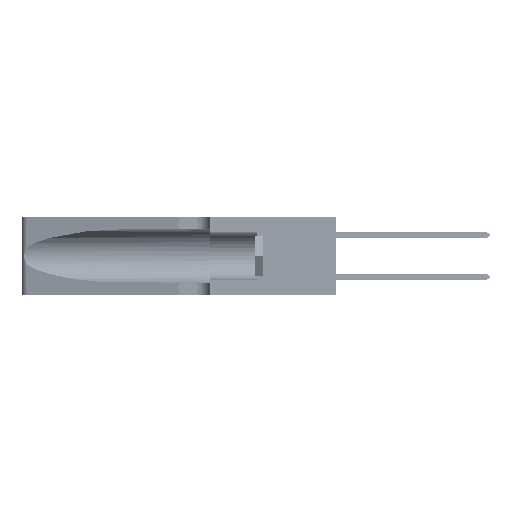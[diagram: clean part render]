
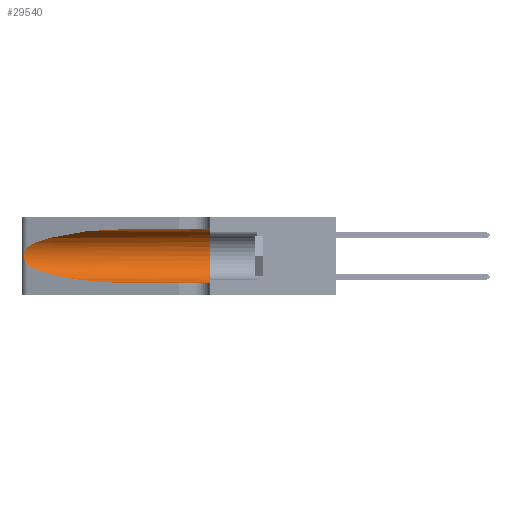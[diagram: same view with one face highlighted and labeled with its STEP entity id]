
A CAD part, left-side view. The second image highlights one B-rep face of the part: STEP entity #29540.
In plain terms, the highlighted cylindrical face has radius 3.308 mm (diameter 6.617 mm), a partial arc.
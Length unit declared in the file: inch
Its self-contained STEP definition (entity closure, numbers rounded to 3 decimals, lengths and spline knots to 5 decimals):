
#598 = FACE_OUTER_BOUND ( 'NONE', #2545, .T. ) ;
#1871 = ORIENTED_EDGE ( 'NONE', *, *, #4116, .T. ) ;
#2001 = CARTESIAN_POINT ( 'NONE',  ( 0.26075, 1.23896, 0.178 ) ) ;
#2328 = CARTESIAN_POINT ( 'NONE',  ( 0.25789, 1.23486, 0.15765 ) ) ;
#2545 = EDGE_LOOP ( 'NONE', ( #1871, #45478, #29068, #12682, #44403, #47040 ) ) ;
#3581 = B_SPLINE_CURVE_WITH_KNOTS ( 'NONE', 3,
 ( #9577, #37362, #22028, #49326, #21513, #45656, #10251, #2001, #37871, #29600, #2328, #5927, #49850, #9922 ),
 .UNSPECIFIED., .F., .F.,
 ( 4, 2, 2, 2, 2, 2, 4 ),
 ( 0., 0.00027, 0.00053, 0.00107, 0.0016, 0.00187, 0.00214 ),
 .UNSPECIFIED. ) ;
#4116 = EDGE_CURVE ( 'NONE', #36163, #9208, #4885, .T. ) ;
#4885 =( BOUNDED_CURVE ( )  B_SPLINE_CURVE ( 3, ( #5275, #32957, #40809, #21198 ),
 .UNSPECIFIED., .F., .F. ) 
 B_SPLINE_CURVE_WITH_KNOTS ( ( 4, 4 ),
 ( 1.5708, 2.84003 ),
 .UNSPECIFIED. ) 
 CURVE ( )  GEOMETRIC_REPRESENTATION_ITEM ( )  RATIONAL_B_SPLINE_CURVE ( ( 1., 0.87, 0.87, 1. ) ) 
 REPRESENTATION_ITEM ( '' )  );
#5275 = CARTESIAN_POINT ( 'NONE',  ( 0.1305, 0.72297, 0.31525 ) ) ;
#5927 = CARTESIAN_POINT ( 'NONE',  ( 0.25639, 1.23186, 0.15144 ) ) ;
#6183 = VECTOR ( 'NONE', #44947, 39.37008 ) ;
#6485 = DIRECTION ( 'NONE',  ( 0., -1., 0. ) ) ;
#7866 = CARTESIAN_POINT ( 'NONE',  ( 0.18966, 0.96281, 0.05475 ) ) ;
#7978 = DIRECTION ( 'NONE',  ( 0., 0., -1. ) ) ;
#8388 = CARTESIAN_POINT ( 'NONE',  ( 0.1305, 0.72297, 0.05475 ) ) ;
#8554 = CARTESIAN_POINT ( 'NONE',  ( 0.2373, 1.15595, 0.08982 ) ) ;
#9208 = VERTEX_POINT ( 'NONE', #44152 ) ;
#9269 = AXIS2_PLACEMENT_3D ( 'NONE', #34825, #50746, #35329 ) ;
#9577 = CARTESIAN_POINT ( 'NONE',  ( 0.25487, 1.22718, 0.22369 ) ) ;
#9922 = CARTESIAN_POINT ( 'NONE',  ( 0.25487, 1.22718, 0.14631 ) ) ;
#10251 = CARTESIAN_POINT ( 'NONE',  ( 0.26075, 1.23896, 0.19203 ) ) ;
#10557 = LINE ( 'NONE', #17931, #45785 ) ;
#12682 = ORIENTED_EDGE ( 'NONE', *, *, #26631, .T. ) ;
#16242 = CARTESIAN_POINT ( 'NONE',  ( 0.1305, 0.35, 0.05475 ) ) ;
#16866 = AXIS2_PLACEMENT_3D ( 'NONE', #23728, #47552, #7978 ) ;
#17245 = CARTESIAN_POINT ( 'NONE',  ( 0.1305, 0.35, 0.31525 ) ) ;
#17931 = CARTESIAN_POINT ( 'NONE',  ( 0.1305, 1.61858, 0.31525 ) ) ;
#19956 = EDGE_CURVE ( 'NONE', #27163, #28211, #43864, .T. ) ;
#20347 = CARTESIAN_POINT ( 'NONE',  ( 0.25487, 1.22718, 0.14631 ) ) ;
#21198 = CARTESIAN_POINT ( 'NONE',  ( 0.25487, 1.22718, 0.22369 ) ) ;
#21513 = CARTESIAN_POINT ( 'NONE',  ( 0.25854, 1.2359, 0.20912 ) ) ;
#22028 = CARTESIAN_POINT ( 'NONE',  ( 0.25639, 1.23184, 0.21858 ) ) ;
#22654 = VERTEX_POINT ( 'NONE', #30158 ) ;
#23728 = CARTESIAN_POINT ( 'NONE',  ( 0.1305, 1.61858, 0.185 ) ) ;
#26631 = EDGE_CURVE ( 'NONE', #33706, #28211, #37057, .T. ) ;
#27163 = VERTEX_POINT ( 'NONE', #17245 ) ;
#28211 = VERTEX_POINT ( 'NONE', #16242 ) ;
#29068 = ORIENTED_EDGE ( 'NONE', *, *, #49940, .T. ) ;
#29540 = ADVANCED_FACE ( 'NONE', ( #598 ), #35200, .F. ) ;
#29600 = CARTESIAN_POINT ( 'NONE',  ( 0.25856, 1.23593, 0.16098 ) ) ;
#30158 = CARTESIAN_POINT ( 'NONE',  ( 0.25487, 1.22718, 0.14631 ) ) ;
#32957 = CARTESIAN_POINT ( 'NONE',  ( 0.18966, 0.96281, 0.31525 ) ) ;
#33706 = VERTEX_POINT ( 'NONE', #34232 ) ;
#34232 = CARTESIAN_POINT ( 'NONE',  ( 0.1305, 0.72297, 0.05475 ) ) ;
#34825 = CARTESIAN_POINT ( 'NONE',  ( 0.1305, 0.35, 0.185 ) ) ;
#34956 = CARTESIAN_POINT ( 'NONE',  ( 0.1305, 1.61858, 0.05475 ) ) ;
#35200 = CYLINDRICAL_SURFACE ( 'NONE', #16866, 0.13025 ) ;
#35329 = DIRECTION ( 'NONE',  ( 0., 0., 1. ) ) ;
#36163 = VERTEX_POINT ( 'NONE', #50884 ) ;
#37057 = LINE ( 'NONE', #34956, #6183 ) ;
#37362 = CARTESIAN_POINT ( 'NONE',  ( 0.25555, 1.22994, 0.2215 ) ) ;
#37871 = CARTESIAN_POINT ( 'NONE',  ( 0.26017, 1.23833, 0.17102 ) ) ;
#40809 = CARTESIAN_POINT ( 'NONE',  ( 0.2373, 1.15595, 0.28018 ) ) ;
#42547 = EDGE_CURVE ( 'NONE', #9208, #22654, #3581, .T. ) ;
#43864 = CIRCLE ( 'NONE', #9269, 0.13025 ) ;
#43981 = EDGE_CURVE ( 'NONE', #36163, #27163, #10557, .T. ) ;
#44152 = CARTESIAN_POINT ( 'NONE',  ( 0.25487, 1.22718, 0.22369 ) ) ;
#44403 = ORIENTED_EDGE ( 'NONE', *, *, #19956, .F. ) ;
#44947 = DIRECTION ( 'NONE',  ( 0., -1., 0. ) ) ;
#45478 = ORIENTED_EDGE ( 'NONE', *, *, #42547, .T. ) ;
#45656 = CARTESIAN_POINT ( 'NONE',  ( 0.26018, 1.23835, 0.19895 ) ) ;
#45785 = VECTOR ( 'NONE', #6485, 39.37008 ) ;
#47040 = ORIENTED_EDGE ( 'NONE', *, *, #43981, .F. ) ;
#47552 = DIRECTION ( 'NONE',  ( 0., -1., 0. ) ) ;
#49326 = CARTESIAN_POINT ( 'NONE',  ( 0.25787, 1.23484, 0.2124 ) ) ;
#49850 = CARTESIAN_POINT ( 'NONE',  ( 0.25555, 1.22993, 0.14849 ) ) ;
#49940 = EDGE_CURVE ( 'NONE', #22654, #33706, #50195, .T. ) ;
#50195 =( BOUNDED_CURVE ( )  B_SPLINE_CURVE ( 3, ( #20347, #8554, #7866, #8388 ),
 .UNSPECIFIED., .F., .T. ) 
 B_SPLINE_CURVE_WITH_KNOTS ( ( 4, 4 ),
 ( 3.44316, 4.71239 ),
 .UNSPECIFIED. ) 
 CURVE ( )  GEOMETRIC_REPRESENTATION_ITEM ( )  RATIONAL_B_SPLINE_CURVE ( ( 1., 0.87, 0.87, 1. ) ) 
 REPRESENTATION_ITEM ( '' )  );
#50746 = DIRECTION ( 'NONE',  ( 0., 1., 0. ) ) ;
#50884 = CARTESIAN_POINT ( 'NONE',  ( 0.1305, 0.72297, 0.31525 ) ) ;
